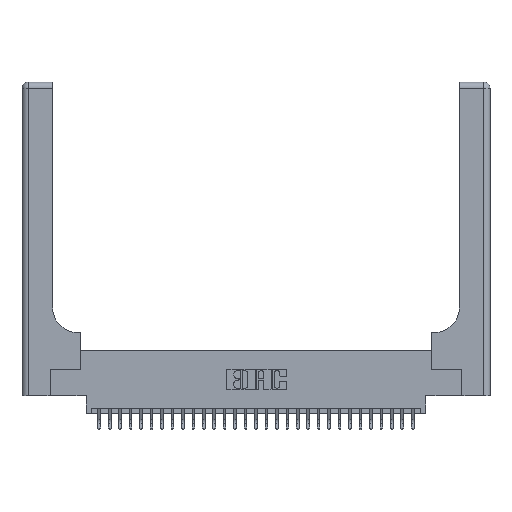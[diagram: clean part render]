
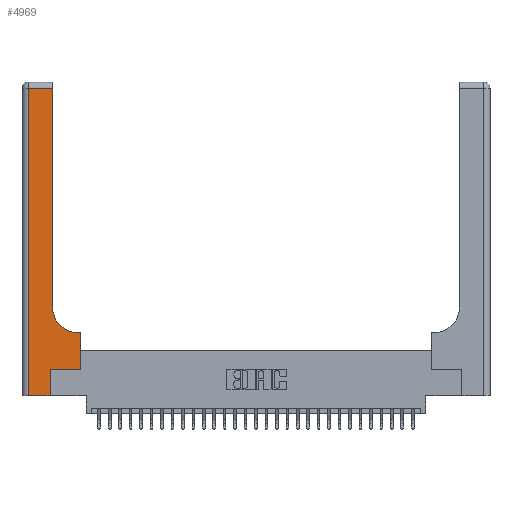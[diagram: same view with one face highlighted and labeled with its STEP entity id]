
A CAD part, top view. The second image highlights one B-rep face of the part: STEP entity #4969.
In plain terms, the highlighted planar face has unit normal (0, 0, 1).
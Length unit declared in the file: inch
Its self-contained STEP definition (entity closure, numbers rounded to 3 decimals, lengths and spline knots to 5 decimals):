
#298 = CARTESIAN_POINT ( 'NONE',  ( 0.2915, 0.85, 0.37 ) ) ;
#359 = CARTESIAN_POINT ( 'NONE',  ( 0.2915, 0.6, 0.37 ) ) ;
#1117 = DIRECTION ( 'NONE',  ( 0., 0., -1. ) ) ;
#1690 = VERTEX_POINT ( 'NONE', #12781 ) ;
#1949 = EDGE_CURVE ( 'NONE', #26512, #22850, #16674, .T. ) ;
#2156 = DIRECTION ( 'NONE',  ( 1., 0., 0. ) ) ;
#2300 = VERTEX_POINT ( 'NONE', #21824 ) ;
#3115 = CARTESIAN_POINT ( 'NONE',  ( 0.269, 0., 0.37 ) ) ;
#3406 = EDGE_CURVE ( 'NONE', #19387, #26512, #8733, .T. ) ;
#4254 = EDGE_CURVE ( 'NONE', #17202, #26394, #9462, .T. ) ;
#4969 = ADVANCED_FACE ( 'NONE', ( #9032 ), #15872, .F. ) ;
#5258 = CARTESIAN_POINT ( 'NONE',  ( 0., 2.94, 0.37 ) ) ;
#5593 = EDGE_CURVE ( 'NONE', #11290, #1690, #10901, .T. ) ;
#5969 = EDGE_CURVE ( 'NONE', #14048, #11290, #20360, .T. ) ;
#6987 = LINE ( 'NONE', #8811, #24087 ) ;
#7071 = ORIENTED_EDGE ( 'NONE', *, *, #4254, .T. ) ;
#7106 = LINE ( 'NONE', #23453, #19365 ) ;
#8272 = VECTOR ( 'NONE', #2156, 39.37008 ) ;
#8355 = DIRECTION ( 'NONE',  ( 0., 0., -1. ) ) ;
#8452 = CARTESIAN_POINT ( 'NONE',  ( 0., 3., 0.37 ) ) ;
#8605 = CARTESIAN_POINT ( 'NONE',  ( 0.5415, 0.6, 0.37 ) ) ;
#8733 = LINE ( 'NONE', #359, #26470 ) ;
#8811 = CARTESIAN_POINT ( 'NONE',  ( 0.2915, 3., 0.37 ) ) ;
#8837 = ORIENTED_EDGE ( 'NONE', *, *, #18756, .T. ) ;
#8988 = DIRECTION ( 'NONE',  ( 0., -1., 0. ) ) ;
#9032 = FACE_OUTER_BOUND ( 'NONE', #25592, .T. ) ;
#9462 = LINE ( 'NONE', #27505, #27920 ) ;
#9840 = CARTESIAN_POINT ( 'NONE',  ( 0.06, 2.94, 0.37 ) ) ;
#10875 = ORIENTED_EDGE ( 'NONE', *, *, #1949, .T. ) ;
#10901 = LINE ( 'NONE', #11456, #29312 ) ;
#10954 = ORIENTED_EDGE ( 'NONE', *, *, #5593, .T. ) ;
#11290 = VERTEX_POINT ( 'NONE', #9840 ) ;
#11456 = CARTESIAN_POINT ( 'NONE',  ( 0.06, 3., 0.37 ) ) ;
#12781 = CARTESIAN_POINT ( 'NONE',  ( 0.06, 0., 0.37 ) ) ;
#13774 = ORIENTED_EDGE ( 'NONE', *, *, #18592, .T. ) ;
#14048 = VERTEX_POINT ( 'NONE', #16741 ) ;
#15872 = PLANE ( 'NONE',  #17282 ) ;
#16315 = EDGE_CURVE ( 'NONE', #2300, #19387, #30649, .T. ) ;
#16674 = CIRCLE ( 'NONE', #19452, 0.25 ) ;
#16741 = CARTESIAN_POINT ( 'NONE',  ( 0.2915, 2.94, 0.37 ) ) ;
#17202 = VERTEX_POINT ( 'NONE', #3115 ) ;
#17282 = AXIS2_PLACEMENT_3D ( 'NONE', #8452, #1117, #18298 ) ;
#17912 = CARTESIAN_POINT ( 'NONE',  ( 0.269, 0.25, 0.37 ) ) ;
#18018 = DIRECTION ( 'NONE',  ( 0., 1., 0. ) ) ;
#18298 = DIRECTION ( 'NONE',  ( -1., 0., 0. ) ) ;
#18592 = EDGE_CURVE ( 'NONE', #26394, #2300, #7106, .T. ) ;
#18756 = EDGE_CURVE ( 'NONE', #1690, #17202, #27553, .T. ) ;
#19365 = VECTOR ( 'NONE', #25851, 39.37008 ) ;
#19387 = VERTEX_POINT ( 'NONE', #24250 ) ;
#19452 = AXIS2_PLACEMENT_3D ( 'NONE', #22882, #8355, #25272 ) ;
#19627 = VECTOR ( 'NONE', #19922, 39.37008 ) ;
#19922 = DIRECTION ( 'NONE',  ( -1., 0., 0. ) ) ;
#19957 = DIRECTION ( 'NONE',  ( -1., 0., 0. ) ) ;
#20360 = LINE ( 'NONE', #5258, #19627 ) ;
#21174 = EDGE_CURVE ( 'NONE', #22850, #14048, #6987, .T. ) ;
#21179 = ORIENTED_EDGE ( 'NONE', *, *, #21174, .T. ) ;
#21824 = CARTESIAN_POINT ( 'NONE',  ( 0.5585, 0.25, 0.37 ) ) ;
#22850 = VERTEX_POINT ( 'NONE', #298 ) ;
#22869 = ORIENTED_EDGE ( 'NONE', *, *, #3406, .T. ) ;
#22882 = CARTESIAN_POINT ( 'NONE',  ( 0.5415, 0.85, 0.37 ) ) ;
#23379 = ORIENTED_EDGE ( 'NONE', *, *, #16315, .T. ) ;
#23453 = CARTESIAN_POINT ( 'NONE',  ( 0.269, 0.25, 0.37 ) ) ;
#23696 = DIRECTION ( 'NONE',  ( 0., 1., 0. ) ) ;
#24020 = ORIENTED_EDGE ( 'NONE', *, *, #5969, .T. ) ;
#24087 = VECTOR ( 'NONE', #28100, 39.37008 ) ;
#24250 = CARTESIAN_POINT ( 'NONE',  ( 0.5585, 0.6, 0.37 ) ) ;
#25272 = DIRECTION ( 'NONE',  ( 1., 0., 0. ) ) ;
#25592 = EDGE_LOOP ( 'NONE', ( #21179, #24020, #10954, #8837, #7071, #13774, #23379, #22869, #10875 ) ) ;
#25851 = DIRECTION ( 'NONE',  ( 1., 0., 0. ) ) ;
#26394 = VERTEX_POINT ( 'NONE', #17912 ) ;
#26470 = VECTOR ( 'NONE', #19957, 39.37008 ) ;
#26512 = VERTEX_POINT ( 'NONE', #8605 ) ;
#27505 = CARTESIAN_POINT ( 'NONE',  ( 0.269, 0., 0.37 ) ) ;
#27553 = LINE ( 'NONE', #31120, #8272 ) ;
#27920 = VECTOR ( 'NONE', #18018, 39.37008 ) ;
#28100 = DIRECTION ( 'NONE',  ( 0., 1., 0. ) ) ;
#28390 = CARTESIAN_POINT ( 'NONE',  ( 0.5585, 0.25, 0.37 ) ) ;
#29312 = VECTOR ( 'NONE', #8988, 39.37008 ) ;
#29906 = VECTOR ( 'NONE', #23696, 39.37008 ) ;
#30649 = LINE ( 'NONE', #28390, #29906 ) ;
#31120 = CARTESIAN_POINT ( 'NONE',  ( 0., 0., 0.37 ) ) ;
